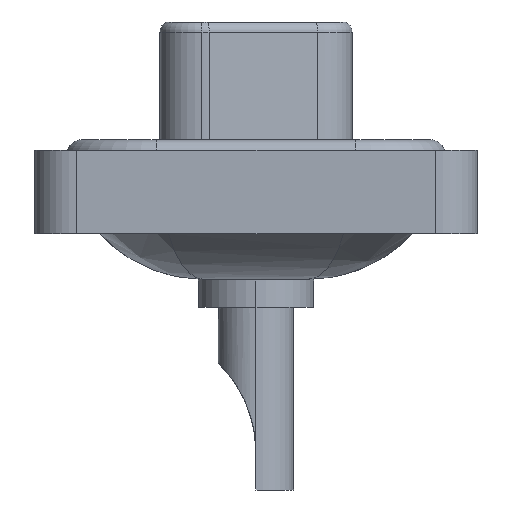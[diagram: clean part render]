
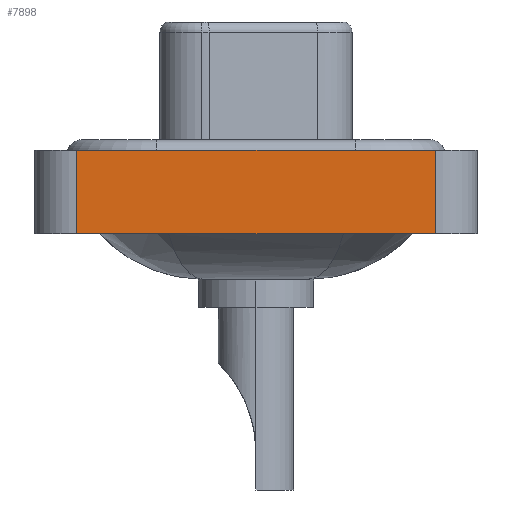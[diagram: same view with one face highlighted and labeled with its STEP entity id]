
A CAD part, left-side view. The second image highlights one B-rep face of the part: STEP entity #7898.
In plain terms, the highlighted planar face has unit normal (-1, 0, 0).
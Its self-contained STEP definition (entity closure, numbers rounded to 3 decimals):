
#159 = VECTOR ( 'NONE', #17570, 1000. ) ;
#288 = EDGE_CURVE ( 'NONE', #12199, #728, #4969, .T. ) ;
#294 = ORIENTED_EDGE ( 'NONE', *, *, #14161, .F. ) ;
#711 = DIRECTION ( 'NONE',  ( 0., -1., 0. ) ) ;
#728 = VERTEX_POINT ( 'NONE', #8555 ) ;
#1827 = CARTESIAN_POINT ( 'NONE',  ( -7.25, 8.55, -3.6 ) ) ;
#3317 = AXIS2_PLACEMENT_3D ( 'NONE', #5076, #3719, #10720 ) ;
#3424 = EDGE_CURVE ( 'NONE', #3864, #13933, #12266, .T. ) ;
#3719 = DIRECTION ( 'NONE',  ( -1., 0., 0. ) ) ;
#3864 = VERTEX_POINT ( 'NONE', #16712 ) ;
#4969 = LINE ( 'NONE', #5059, #159 ) ;
#5059 = CARTESIAN_POINT ( 'NONE',  ( -7.25, 8.55, -3.6 ) ) ;
#5076 = CARTESIAN_POINT ( 'NONE',  ( -7.25, -8.55, -3.6 ) ) ;
#5250 = CARTESIAN_POINT ( 'NONE',  ( -7.25, -8.55, 0.4 ) ) ;
#6455 = FACE_OUTER_BOUND ( 'NONE', #12404, .T. ) ;
#6632 = VECTOR ( 'NONE', #711, 1000. ) ;
#7898 = ADVANCED_FACE ( 'NONE', ( #6455 ), #12081, .T. ) ;
#8518 = DIRECTION ( 'NONE',  ( 0., -1., 0. ) ) ;
#8555 = CARTESIAN_POINT ( 'NONE',  ( -7.25, 8.55, 0.4 ) ) ;
#9641 = LINE ( 'NONE', #16595, #10540 ) ;
#10540 = VECTOR ( 'NONE', #8518, 1000. ) ;
#10720 = DIRECTION ( 'NONE',  ( 0., 0., 1. ) ) ;
#10809 = CARTESIAN_POINT ( 'NONE',  ( -7.25, -8.55, -3.6 ) ) ;
#10968 = VECTOR ( 'NONE', #16377, 1000. ) ;
#11045 = ORIENTED_EDGE ( 'NONE', *, *, #12987, .T. ) ;
#12081 = PLANE ( 'NONE',  #3317 ) ;
#12199 = VERTEX_POINT ( 'NONE', #1827 ) ;
#12266 = LINE ( 'NONE', #10809, #10968 ) ;
#12404 = EDGE_LOOP ( 'NONE', ( #16580, #294, #14381, #11045 ) ) ;
#12987 = EDGE_CURVE ( 'NONE', #12199, #3864, #9641, .T. ) ;
#13496 = LINE ( 'NONE', #14768, #6632 ) ;
#13933 = VERTEX_POINT ( 'NONE', #5250 ) ;
#14161 = EDGE_CURVE ( 'NONE', #728, #13933, #13496, .T. ) ;
#14381 = ORIENTED_EDGE ( 'NONE', *, *, #288, .F. ) ;
#14768 = CARTESIAN_POINT ( 'NONE',  ( -7.25, -8.55, 0.4 ) ) ;
#16377 = DIRECTION ( 'NONE',  ( 0., 0., 1. ) ) ;
#16580 = ORIENTED_EDGE ( 'NONE', *, *, #3424, .T. ) ;
#16595 = CARTESIAN_POINT ( 'NONE',  ( -7.25, -8.55, -3.6 ) ) ;
#16712 = CARTESIAN_POINT ( 'NONE',  ( -7.25, -8.55, -3.6 ) ) ;
#17570 = DIRECTION ( 'NONE',  ( 0., 0., 1. ) ) ;
